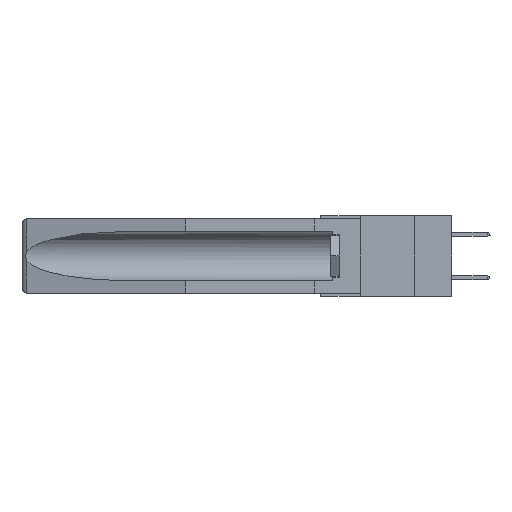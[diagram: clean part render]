
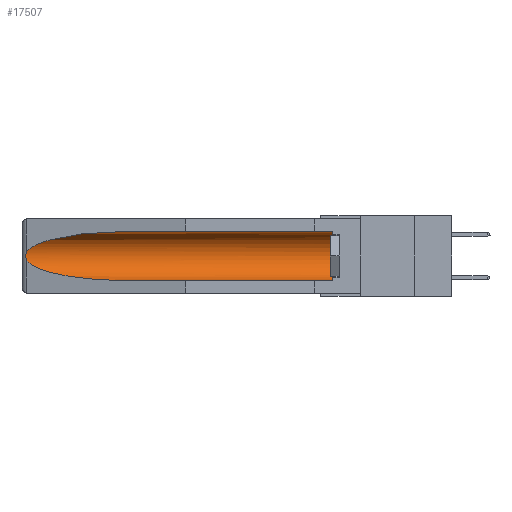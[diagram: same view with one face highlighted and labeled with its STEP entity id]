
A CAD part, left-side view. The second image highlights one B-rep face of the part: STEP entity #17507.
In plain terms, the highlighted cylindrical face has radius 2.857 mm (diameter 5.715 mm), a partial arc.
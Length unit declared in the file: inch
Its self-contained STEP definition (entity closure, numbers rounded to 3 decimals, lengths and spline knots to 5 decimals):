
#382 = CARTESIAN_POINT ( 'NONE',  ( 0.26537, 1.52718, -0.19328 ) ) ;
#675 = VERTEX_POINT ( 'NONE', #14157 ) ;
#722 = CARTESIAN_POINT ( 'NONE',  ( 0.26537, 1.52718, -0.14972 ) ) ;
#792 = VERTEX_POINT ( 'NONE', #4142 ) ;
#981 = CIRCLE ( 'NONE', #8756, 0.1125 ) ;
#1477 = EDGE_LOOP ( 'NONE', ( #11276, #13305, #18121, #5572, #9623, #18002 ) ) ;
#2011 = LINE ( 'NONE', #3710, #15169 ) ;
#2348 = CARTESIAN_POINT ( 'NONE',  ( 0.155, 0.126, -0.284 ) ) ;
#2625 = CYLINDRICAL_SURFACE ( 'NONE', #7175, 0.1125 ) ;
#2720 = CARTESIAN_POINT ( 'NONE',  ( 0.2675, 1.53308, -0.17534 ) ) ;
#2785 = CARTESIAN_POINT ( 'NONE',  ( 0.26537, 1.52718, -0.19328 ) ) ;
#3374 = CARTESIAN_POINT ( 'NONE',  ( 0.155, 1.07973, -0.284 ) ) ;
#3541 = VECTOR ( 'NONE', #8345, 39.37008 ) ;
#3557 = FACE_OUTER_BOUND ( 'NONE', #1477, .T. ) ;
#3710 = CARTESIAN_POINT ( 'NONE',  ( 0.155, -0.30754, -0.059 ) ) ;
#4142 = CARTESIAN_POINT ( 'NONE',  ( 0.155, 1.07973, -0.284 ) ) ;
#5572 = ORIENTED_EDGE ( 'NONE', *, *, #17767, .F. ) ;
#5730 = CARTESIAN_POINT ( 'NONE',  ( 0.2673, 1.5327, -0.16383 ) ) ;
#5783 = CARTESIAN_POINT ( 'NONE',  ( 0.2675, 1.53308, -0.16763 ) ) ;
#5855 = CARTESIAN_POINT ( 'NONE',  ( 0.26597, 1.5296, -0.19026 ) ) ;
#6108 = LINE ( 'NONE', #17322, #3541 ) ;
#6995 = CARTESIAN_POINT ( 'NONE',  ( 0.21114, 1.30732, -0.059 ) ) ;
#7175 = AXIS2_PLACEMENT_3D ( 'NONE', #14413, #11771, #18318 ) ;
#7327 = CARTESIAN_POINT ( 'NONE',  ( 0.26654, 1.53092, -0.15636 ) ) ;
#7535 = EDGE_CURVE ( 'NONE', #14778, #675, #17831, .T. ) ;
#8345 = DIRECTION ( 'NONE',  ( 0., 1., 0. ) ) ;
#8415 = EDGE_CURVE ( 'NONE', #8599, #18839, #2011, .T. ) ;
#8599 = VERTEX_POINT ( 'NONE', #10397 ) ;
#8756 = AXIS2_PLACEMENT_3D ( 'NONE', #15969, #10135, #17349 ) ;
#9239 = EDGE_CURVE ( 'NONE', #675, #792, #16396, .T. ) ;
#9623 = ORIENTED_EDGE ( 'NONE', *, *, #14349, .T. ) ;
#10135 = DIRECTION ( 'NONE',  ( 0., -1., 0. ) ) ;
#10139 = DIRECTION ( 'NONE',  ( 0., 1., 0. ) ) ;
#10319 = CARTESIAN_POINT ( 'NONE',  ( 0.26655, 1.53094, -0.18657 ) ) ;
#10397 = CARTESIAN_POINT ( 'NONE',  ( 0.155, 0.126, -0.059 ) ) ;
#11276 = ORIENTED_EDGE ( 'NONE', *, *, #18955, .T. ) ;
#11771 = DIRECTION ( 'NONE',  ( 0., 1., 0. ) ) ;
#12800 = CARTESIAN_POINT ( 'NONE',  ( 0.25451, 1.48313, -0.09465 ) ) ;
#13085 = CARTESIAN_POINT ( 'NONE',  ( 0.26537, 1.52718, -0.14972 ) ) ;
#13305 = ORIENTED_EDGE ( 'NONE', *, *, #7535, .T. ) ;
#13839 = CARTESIAN_POINT ( 'NONE',  ( 0.25451, 1.48313, -0.24835 ) ) ;
#14157 = CARTESIAN_POINT ( 'NONE',  ( 0.26537, 1.52718, -0.19328 ) ) ;
#14257 = CARTESIAN_POINT ( 'NONE',  ( 0.26537, 1.52718, -0.14972 ) ) ;
#14349 = EDGE_CURVE ( 'NONE', #14617, #8599, #981, .T. ) ;
#14413 = CARTESIAN_POINT ( 'NONE',  ( 0.155, -0.30754, -0.1715 ) ) ;
#14607 =( BOUNDED_CURVE ( )  B_SPLINE_CURVE ( 3, ( #15813, #6995, #12800, #14257 ),
 .UNSPECIFIED., .F., .F. ) 
 B_SPLINE_CURVE_WITH_KNOTS ( ( 4, 4 ),
 ( 4.71239, 6.08839 ),
 .UNSPECIFIED. ) 
 CURVE ( )  GEOMETRIC_REPRESENTATION_ITEM ( )  RATIONAL_B_SPLINE_CURVE ( ( 1., 0.848, 0.848, 1. ) ) 
 REPRESENTATION_ITEM ( '' )  );
#14617 = VERTEX_POINT ( 'NONE', #2348 ) ;
#14660 = CARTESIAN_POINT ( 'NONE',  ( 0.26597, 1.52961, -0.15275 ) ) ;
#14778 = VERTEX_POINT ( 'NONE', #722 ) ;
#15169 = VECTOR ( 'NONE', #10139, 39.37008 ) ;
#15363 = CARTESIAN_POINT ( 'NONE',  ( 0.155, 1.07973, -0.059 ) ) ;
#15813 = CARTESIAN_POINT ( 'NONE',  ( 0.155, 1.07973, -0.059 ) ) ;
#15969 = CARTESIAN_POINT ( 'NONE',  ( 0.155, 0.126, -0.1715 ) ) ;
#16031 = CARTESIAN_POINT ( 'NONE',  ( 0.2673, 1.53269, -0.17917 ) ) ;
#16396 =( BOUNDED_CURVE ( )  B_SPLINE_CURVE ( 3, ( #382, #13839, #18199, #3374 ),
 .UNSPECIFIED., .F., .F. ) 
 B_SPLINE_CURVE_WITH_KNOTS ( ( 4, 4 ),
 ( 0.1948, 1.5708 ),
 .UNSPECIFIED. ) 
 CURVE ( )  GEOMETRIC_REPRESENTATION_ITEM ( )  RATIONAL_B_SPLINE_CURVE ( ( 1., 0.848, 0.848, 1. ) ) 
 REPRESENTATION_ITEM ( '' )  );
#17322 = CARTESIAN_POINT ( 'NONE',  ( 0.155, -0.30754, -0.284 ) ) ;
#17349 = DIRECTION ( 'NONE',  ( 0., 0., 1. ) ) ;
#17507 = ADVANCED_FACE ( 'NONE', ( #3557 ), #2625, .F. ) ;
#17767 = EDGE_CURVE ( 'NONE', #14617, #792, #6108, .T. ) ;
#17831 = B_SPLINE_CURVE_WITH_KNOTS ( 'NONE', 3,
 ( #13085, #14660, #7327, #5730, #5783, #2720, #16031, #10319, #5855, #2785 ),
 .UNSPECIFIED., .F., .F.,
 ( 4, 2, 2, 2, 4 ),
 ( 0., 0.00029, 0.00058, 0.00087, 0.00117 ),
 .UNSPECIFIED. ) ;
#18002 = ORIENTED_EDGE ( 'NONE', *, *, #8415, .T. ) ;
#18121 = ORIENTED_EDGE ( 'NONE', *, *, #9239, .T. ) ;
#18199 = CARTESIAN_POINT ( 'NONE',  ( 0.21114, 1.30732, -0.284 ) ) ;
#18318 = DIRECTION ( 'NONE',  ( 0., 0., 1. ) ) ;
#18839 = VERTEX_POINT ( 'NONE', #15363 ) ;
#18955 = EDGE_CURVE ( 'NONE', #18839, #14778, #14607, .T. ) ;
